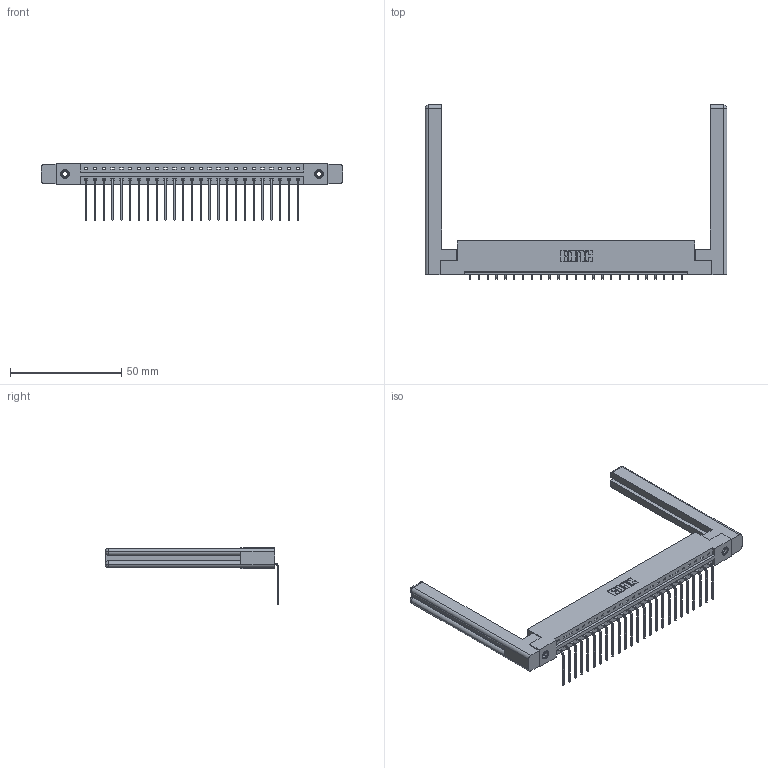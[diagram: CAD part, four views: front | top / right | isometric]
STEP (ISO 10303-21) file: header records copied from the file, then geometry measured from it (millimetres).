
FILE_DESCRIPTION (( 'STEP AP203' ), '1' );
FILE_NAME ('337-025-559-158.STEP', '2019-09-30T18:05:19', ( '' ), ( '' ), 'SwSTEP 2.0', 'SolidWorks 2016', '' );
FILE_SCHEMA (( 'CONFIG_CONTROL_DESIGN' ));
Length unit declared in the file: inch
Products named in the file (5): 337 Part_Flush Mounting Lugs - 0.156 Dia-TI; 345-292-001_558 559 Tail - 1; 307-220-058; 337-025-559-158; 345-250-001_345-250-001-102
Assembly tree (30 placements, depth 2):
  337-025-559-158
    337 Part_Flush Mounting Lugs - 0.156 Dia-TI
    345-292-001_558 559 Tail - 1  x25
    345-250-001_345-250-001-102  x2
    307-220-058  x2
Bounding box: 135.69 x 78.17 x 25.53 mm (x, y, z)
Volume: 21135.1 mm3; surface area: 20069.4 mm2
Topology: 30 solids, 30 shells, 1856 faces, 5515 edges, 3630 vertices
Faces by surface type: plane 1354, cylinder 478, cone 12, torus 12
Entity records: 23500 total; most frequent: CARTESIAN_POINT 4092, ORIENTED_EDGE 3992, DIRECTION 3498, EDGE_CURVE 1996, LINE 1820, VECTOR 1820, VERTEX_POINT 1322, AXIS2_PLACEMENT_3D 839
